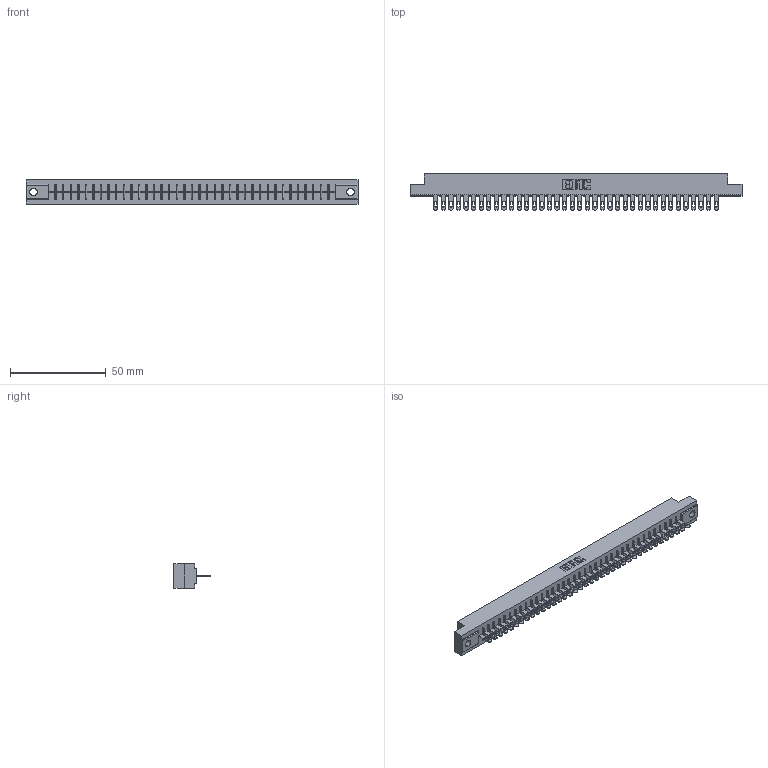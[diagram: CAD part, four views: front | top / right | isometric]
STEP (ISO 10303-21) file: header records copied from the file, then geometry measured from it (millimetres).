
FILE_DESCRIPTION (( 'STEP AP203' ), '1' );
FILE_NAME ('316-038-400-104.STEP', '2020-09-23T05:42:48', ( '' ), ( '' ), 'SwSTEP 2.0', 'SolidWorks 2020', '' );
FILE_SCHEMA (( 'CONFIG_CONTROL_DESIGN' ));
Length unit declared in the file: inch
Products named in the file (3): 306-290-001_100; 316-038-400-104; 306 Part_.156 Dia
Assembly tree (39 placements, depth 2):
  316-038-400-104
    306 Part_.156 Dia
    306-290-001_100  x38
Bounding box: 173.58 x 18.87 x 12.7 mm (x, y, z)
Volume: 19183.4 mm3; surface area: 20120.5 mm2
Topology: 39 solids, 39 shells, 3018 faces, 8522 edges, 5476 vertices
Faces by surface type: plane 1982, cylinder 884, sphere 152
Entity records: 36537 total; most frequent: CARTESIAN_POINT 6139, ORIENTED_EDGE 6084, DIRECTION 6046, EDGE_CURVE 3042, VECTOR 2384, LINE 2384, VERTEX_POINT 1924, AXIS2_PLACEMENT_3D 1831
